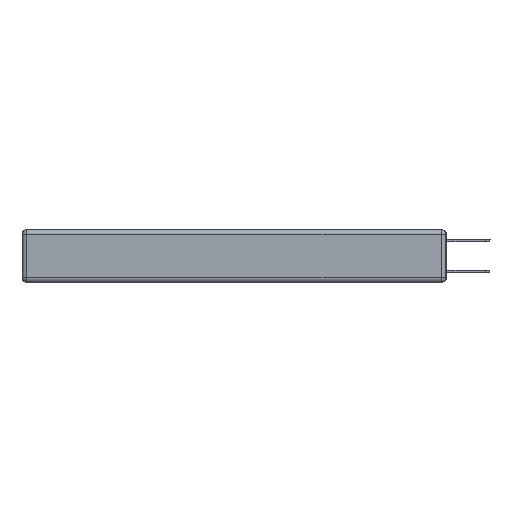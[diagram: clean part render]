
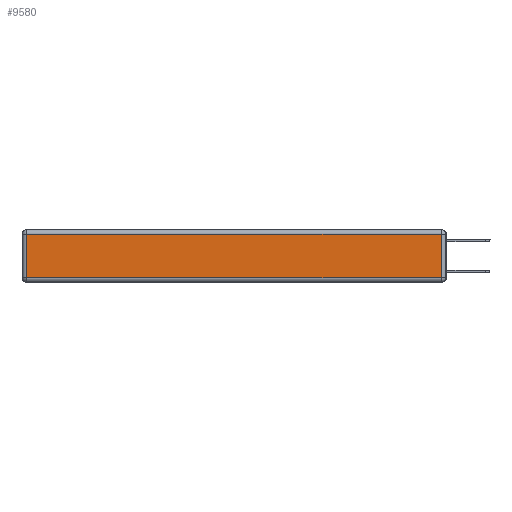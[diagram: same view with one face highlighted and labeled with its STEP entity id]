
A CAD part, left-side view. The second image highlights one B-rep face of the part: STEP entity #9580.
In plain terms, the highlighted planar face has unit normal (-1, 0, 0).
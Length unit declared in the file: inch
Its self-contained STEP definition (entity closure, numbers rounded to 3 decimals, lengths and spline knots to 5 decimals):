
#109 = CARTESIAN_POINT ( 'NONE',  ( 0., 2.72, -0.03 ) ) ;
#757 = ORIENTED_EDGE ( 'NONE', *, *, #13668, .T. ) ;
#996 = CARTESIAN_POINT ( 'NONE',  ( 0., 2.72, -0.343 ) ) ;
#1450 = VECTOR ( 'NONE', #11804, 39.37008 ) ;
#2274 = AXIS2_PLACEMENT_3D ( 'NONE', #10165, #14429, #2512 ) ;
#2512 = DIRECTION ( 'NONE',  ( 0., 0., 1. ) ) ;
#3770 = LINE ( 'NONE', #6797, #17163 ) ;
#4343 = DIRECTION ( 'NONE',  ( 0., 0., 1. ) ) ;
#5943 = EDGE_CURVE ( 'NONE', #11149, #12670, #3770, .T. ) ;
#5965 = ORIENTED_EDGE ( 'NONE', *, *, #16806, .T. ) ;
#6797 = CARTESIAN_POINT ( 'NONE',  ( 0., 0., -0.313 ) ) ;
#6829 = VECTOR ( 'NONE', #4343, 39.37008 ) ;
#7737 = CARTESIAN_POINT ( 'NONE',  ( 0., 2.72, -0.313 ) ) ;
#8405 = PLANE ( 'NONE',  #2274 ) ;
#8659 = CARTESIAN_POINT ( 'NONE',  ( 0., 2.75, -0.03 ) ) ;
#8944 = EDGE_LOOP ( 'NONE', ( #10792, #5965, #757, #13960 ) ) ;
#9580 = ADVANCED_FACE ( 'NONE', ( #17655 ), #8405, .T. ) ;
#9750 = DIRECTION ( 'NONE',  ( 0., -1., 0. ) ) ;
#10165 = CARTESIAN_POINT ( 'NONE',  ( 0., 0., -0.343 ) ) ;
#10343 = CARTESIAN_POINT ( 'NONE',  ( 0., 0.03, -0.03 ) ) ;
#10792 = ORIENTED_EDGE ( 'NONE', *, *, #5943, .T. ) ;
#11149 = VERTEX_POINT ( 'NONE', #7737 ) ;
#11804 = DIRECTION ( 'NONE',  ( 0., 0., -1. ) ) ;
#11826 = CARTESIAN_POINT ( 'NONE',  ( 0., 0.03, -0.343 ) ) ;
#12670 = VERTEX_POINT ( 'NONE', #15038 ) ;
#13215 = DIRECTION ( 'NONE',  ( 0., 1., 0. ) ) ;
#13313 = LINE ( 'NONE', #8659, #18096 ) ;
#13668 = EDGE_CURVE ( 'NONE', #16849, #18733, #13313, .T. ) ;
#13960 = ORIENTED_EDGE ( 'NONE', *, *, #18610, .T. ) ;
#14429 = DIRECTION ( 'NONE',  ( -1., 0., 0. ) ) ;
#15038 = CARTESIAN_POINT ( 'NONE',  ( 0., 0.03, -0.313 ) ) ;
#15972 = LINE ( 'NONE', #11826, #6829 ) ;
#16806 = EDGE_CURVE ( 'NONE', #12670, #16849, #15972, .T. ) ;
#16849 = VERTEX_POINT ( 'NONE', #10343 ) ;
#17163 = VECTOR ( 'NONE', #9750, 39.37008 ) ;
#17655 = FACE_OUTER_BOUND ( 'NONE', #8944, .T. ) ;
#18096 = VECTOR ( 'NONE', #13215, 39.37008 ) ;
#18610 = EDGE_CURVE ( 'NONE', #18733, #11149, #19172, .T. ) ;
#18733 = VERTEX_POINT ( 'NONE', #109 ) ;
#19172 = LINE ( 'NONE', #996, #1450 ) ;
